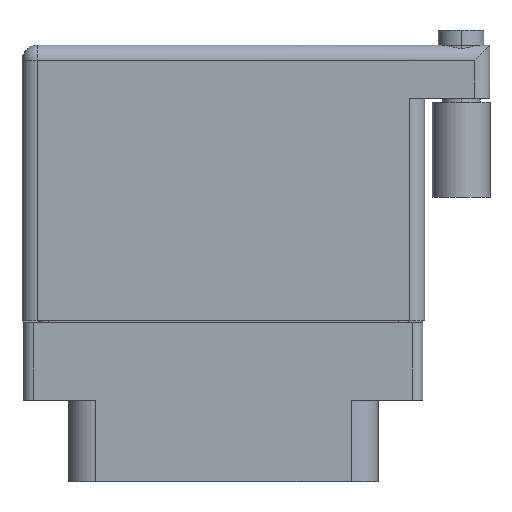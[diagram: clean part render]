
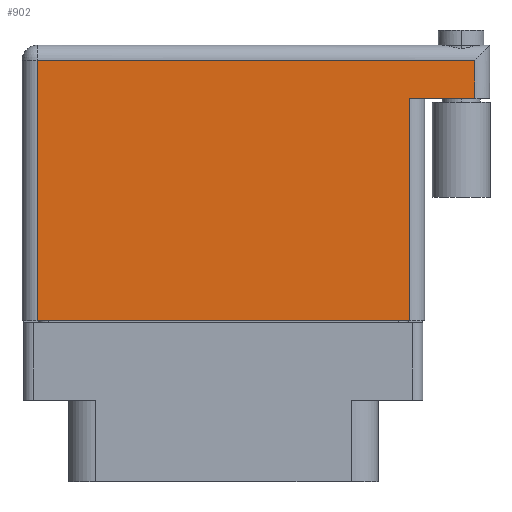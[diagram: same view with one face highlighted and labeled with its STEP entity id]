
A CAD part, front view. The second image highlights one B-rep face of the part: STEP entity #902.
In plain terms, the highlighted face is planar.
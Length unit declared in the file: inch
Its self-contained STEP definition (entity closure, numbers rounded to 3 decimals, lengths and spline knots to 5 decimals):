
#11 = CARTESIAN_POINT ( 'NONE',  ( 0.6125, 0.631, 0.3575 ) ) ;
#902 = ADVANCED_FACE ( 'NONE', ( #17243 ), #2846, .F. ) ;
#1870 = VERTEX_POINT ( 'NONE', #17783 ) ;
#1965 = VECTOR ( 'NONE', #21073, 39.37008 ) ;
#2061 = DIRECTION ( 'NONE',  ( 0., -1., 0. ) ) ;
#2499 = CARTESIAN_POINT ( 'NONE',  ( -0.6125, -0.1, 0.3575 ) ) ;
#2569 = VECTOR ( 'NONE', #21148, 39.37008 ) ;
#2846 = PLANE ( 'NONE',  #11288 ) ;
#3462 = ORIENTED_EDGE ( 'NONE', *, *, #5423, .T. ) ;
#4448 = ORIENTED_EDGE ( 'NONE', *, *, #17816, .T. ) ;
#4640 = VERTEX_POINT ( 'NONE', #11017 ) ;
#4716 = VERTEX_POINT ( 'NONE', #11 ) ;
#5423 = EDGE_CURVE ( 'NONE', #4640, #4716, #13566, .T. ) ;
#5476 = VECTOR ( 'NONE', #9952, 39.37008 ) ;
#6104 = CARTESIAN_POINT ( 'NONE',  ( 0.8265, 0.756, 0.3575 ) ) ;
#6242 = ORIENTED_EDGE ( 'NONE', *, *, #18866, .T. ) ;
#6566 = VERTEX_POINT ( 'NONE', #19135 ) ;
#7258 = VERTEX_POINT ( 'NONE', #6104 ) ;
#7458 = DIRECTION ( 'NONE',  ( -1., 0., 0. ) ) ;
#9040 = CARTESIAN_POINT ( 'NONE',  ( -0.6625, 0.806, 0.3575 ) ) ;
#9952 = DIRECTION ( 'NONE',  ( 0., 1., 0. ) ) ;
#10730 = LINE ( 'NONE', #12845, #12544 ) ;
#10896 = EDGE_CURVE ( 'NONE', #7258, #1870, #14570, .T. ) ;
#10919 = DIRECTION ( 'NONE',  ( 0., 0., -1. ) ) ;
#11017 = CARTESIAN_POINT ( 'NONE',  ( 0.6125, -0.1, 0.3575 ) ) ;
#11264 = LINE ( 'NONE', #21146, #21671 ) ;
#11288 = AXIS2_PLACEMENT_3D ( 'NONE', #9040, #10919, #7458 ) ;
#12544 = VECTOR ( 'NONE', #20874, 39.37008 ) ;
#12724 = CARTESIAN_POINT ( 'NONE',  ( -0.6625, 0.756, 0.3575 ) ) ;
#12796 = EDGE_CURVE ( 'NONE', #6566, #4716, #10730, .T. ) ;
#12845 = CARTESIAN_POINT ( 'NONE',  ( 0.8765, 0.631, 0.3575 ) ) ;
#13152 = VERTEX_POINT ( 'NONE', #2499 ) ;
#13566 = LINE ( 'NONE', #17636, #1965 ) ;
#13872 = ORIENTED_EDGE ( 'NONE', *, *, #10896, .T. ) ;
#14570 = LINE ( 'NONE', #12724, #2569 ) ;
#17243 = FACE_OUTER_BOUND ( 'NONE', #20735, .T. ) ;
#17610 = LINE ( 'NONE', #19981, #5476 ) ;
#17636 = CARTESIAN_POINT ( 'NONE',  ( 0.6125, 0.631, 0.3575 ) ) ;
#17783 = CARTESIAN_POINT ( 'NONE',  ( -0.6125, 0.756, 0.3575 ) ) ;
#17816 = EDGE_CURVE ( 'NONE', #13152, #4640, #11264, .T. ) ;
#18866 = EDGE_CURVE ( 'NONE', #6566, #7258, #17610, .T. ) ;
#18915 = DIRECTION ( 'NONE',  ( 1., 0., 0. ) ) ;
#19135 = CARTESIAN_POINT ( 'NONE',  ( 0.8265, 0.631, 0.3575 ) ) ;
#19883 = LINE ( 'NONE', #23828, #21674 ) ;
#19981 = CARTESIAN_POINT ( 'NONE',  ( 0.8265, 0.806, 0.3575 ) ) ;
#20735 = EDGE_LOOP ( 'NONE', ( #4448, #3462, #25567, #6242, #13872, #23970 ) ) ;
#20874 = DIRECTION ( 'NONE',  ( -1., 0., 0. ) ) ;
#21073 = DIRECTION ( 'NONE',  ( 0., 1., 0. ) ) ;
#21146 = CARTESIAN_POINT ( 'NONE',  ( -0.6625, -0.1, 0.3575 ) ) ;
#21148 = DIRECTION ( 'NONE',  ( -1., 0., 0. ) ) ;
#21671 = VECTOR ( 'NONE', #18915, 39.37008 ) ;
#21674 = VECTOR ( 'NONE', #2061, 39.37008 ) ;
#22577 = EDGE_CURVE ( 'NONE', #1870, #13152, #19883, .T. ) ;
#23828 = CARTESIAN_POINT ( 'NONE',  ( -0.6125, -0.1, 0.3575 ) ) ;
#23970 = ORIENTED_EDGE ( 'NONE', *, *, #22577, .T. ) ;
#25567 = ORIENTED_EDGE ( 'NONE', *, *, #12796, .F. ) ;
